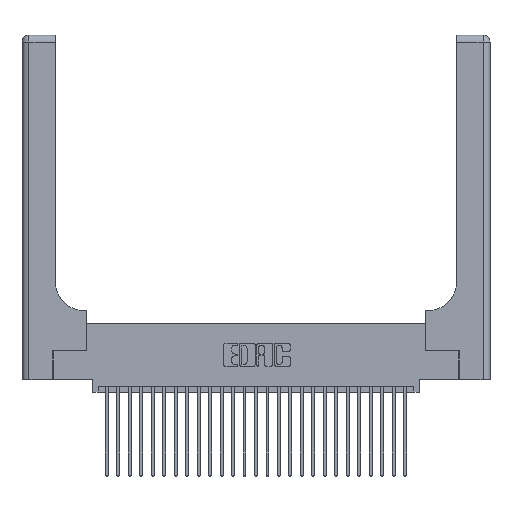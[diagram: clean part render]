
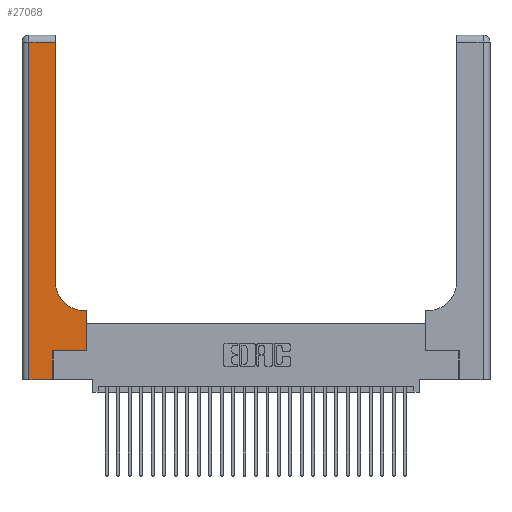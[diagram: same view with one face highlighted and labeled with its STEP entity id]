
A CAD part, top view. The second image highlights one B-rep face of the part: STEP entity #27068.
In plain terms, the highlighted planar face has unit normal (0, 0, 1).
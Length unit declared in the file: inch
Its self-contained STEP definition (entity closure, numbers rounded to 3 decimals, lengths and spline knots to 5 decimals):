
#70 = DIRECTION ( 'NONE',  ( 0., 1., 0. ) ) ;
#232 = DIRECTION ( 'NONE',  ( -1., 0., 0. ) ) ;
#331 = LINE ( 'NONE', #8050, #4463 ) ;
#711 = CARTESIAN_POINT ( 'NONE',  ( 0.2915, 3., 0.37 ) ) ;
#881 = ORIENTED_EDGE ( 'NONE', *, *, #12145, .T. ) ;
#1142 = VERTEX_POINT ( 'NONE', #8361 ) ;
#1199 = VERTEX_POINT ( 'NONE', #6777 ) ;
#1335 = ORIENTED_EDGE ( 'NONE', *, *, #14976, .T. ) ;
#1405 = VERTEX_POINT ( 'NONE', #6571 ) ;
#1464 = ORIENTED_EDGE ( 'NONE', *, *, #23641, .T. ) ;
#1806 = DIRECTION ( 'NONE',  ( 1., 0., 0. ) ) ;
#2013 = CARTESIAN_POINT ( 'NONE',  ( 0.5415, 0.85, 0.37 ) ) ;
#2093 = LINE ( 'NONE', #711, #17286 ) ;
#2987 = ORIENTED_EDGE ( 'NONE', *, *, #19149, .T. ) ;
#3297 = EDGE_CURVE ( 'NONE', #17739, #1199, #13120, .T. ) ;
#3792 = FACE_OUTER_BOUND ( 'NONE', #11331, .T. ) ;
#3968 = VECTOR ( 'NONE', #5839, 39.37008 ) ;
#4463 = VECTOR ( 'NONE', #28068, 39.37008 ) ;
#4515 = CARTESIAN_POINT ( 'NONE',  ( 0.269, 0., 0.37 ) ) ;
#4534 = EDGE_CURVE ( 'NONE', #8665, #1142, #23366, .T. ) ;
#4782 = PLANE ( 'NONE',  #22796 ) ;
#4822 = VECTOR ( 'NONE', #16466, 39.37008 ) ;
#5832 = CARTESIAN_POINT ( 'NONE',  ( 0.2915, 0.6, 0.37 ) ) ;
#5839 = DIRECTION ( 'NONE',  ( -1., 0., 0. ) ) ;
#5978 = VECTOR ( 'NONE', #22544, 39.37008 ) ;
#6223 = LINE ( 'NONE', #26571, #25215 ) ;
#6312 = LINE ( 'NONE', #5832, #12573 ) ;
#6571 = CARTESIAN_POINT ( 'NONE',  ( 0.2915, 2.94, 0.37 ) ) ;
#6777 = CARTESIAN_POINT ( 'NONE',  ( 0.5585, 0.25, 0.37 ) ) ;
#7262 = EDGE_CURVE ( 'NONE', #9841, #19209, #14631, .T. ) ;
#8050 = CARTESIAN_POINT ( 'NONE',  ( 0., 0., 0.37 ) ) ;
#8144 = LINE ( 'NONE', #19486, #3968 ) ;
#8361 = CARTESIAN_POINT ( 'NONE',  ( 0.2915, 0.85, 0.37 ) ) ;
#8665 = VERTEX_POINT ( 'NONE', #24727 ) ;
#8831 = DIRECTION ( 'NONE',  ( 0., 1., 0. ) ) ;
#9298 = AXIS2_PLACEMENT_3D ( 'NONE', #2013, #13096, #1806 ) ;
#9841 = VERTEX_POINT ( 'NONE', #17469 ) ;
#10858 = EDGE_CURVE ( 'NONE', #1405, #9841, #8144, .T. ) ;
#11331 = EDGE_LOOP ( 'NONE', ( #1335, #15556, #21869, #14901, #1464, #16745, #2987, #881, #26623 ) ) ;
#12145 = EDGE_CURVE ( 'NONE', #14466, #8665, #6312, .T. ) ;
#12573 = VECTOR ( 'NONE', #27729, 39.37008 ) ;
#13096 = DIRECTION ( 'NONE',  ( 0., 0., -1. ) ) ;
#13120 = LINE ( 'NONE', #16359, #4822 ) ;
#13189 = CARTESIAN_POINT ( 'NONE',  ( 0.06, 0., 0.37 ) ) ;
#13396 = CARTESIAN_POINT ( 'NONE',  ( 0., 3., 0.37 ) ) ;
#14466 = VERTEX_POINT ( 'NONE', #15961 ) ;
#14631 = LINE ( 'NONE', #18017, #5978 ) ;
#14901 = ORIENTED_EDGE ( 'NONE', *, *, #27447, .T. ) ;
#14976 = EDGE_CURVE ( 'NONE', #1142, #1405, #2093, .T. ) ;
#15240 = CARTESIAN_POINT ( 'NONE',  ( 0.269, 0., 0.37 ) ) ;
#15556 = ORIENTED_EDGE ( 'NONE', *, *, #10858, .T. ) ;
#15611 = DIRECTION ( 'NONE',  ( 0., 0., -1. ) ) ;
#15961 = CARTESIAN_POINT ( 'NONE',  ( 0.5585, 0.6, 0.37 ) ) ;
#16359 = CARTESIAN_POINT ( 'NONE',  ( 0.269, 0.25, 0.37 ) ) ;
#16466 = DIRECTION ( 'NONE',  ( 1., 0., 0. ) ) ;
#16745 = ORIENTED_EDGE ( 'NONE', *, *, #3297, .T. ) ;
#17286 = VECTOR ( 'NONE', #18497, 39.37008 ) ;
#17469 = CARTESIAN_POINT ( 'NONE',  ( 0.06, 2.94, 0.37 ) ) ;
#17739 = VERTEX_POINT ( 'NONE', #19750 ) ;
#18017 = CARTESIAN_POINT ( 'NONE',  ( 0.06, 3., 0.37 ) ) ;
#18497 = DIRECTION ( 'NONE',  ( 0., 1., 0. ) ) ;
#19149 = EDGE_CURVE ( 'NONE', #1199, #14466, #6223, .T. ) ;
#19181 = VECTOR ( 'NONE', #70, 39.37008 ) ;
#19209 = VERTEX_POINT ( 'NONE', #13189 ) ;
#19486 = CARTESIAN_POINT ( 'NONE',  ( 0., 2.94, 0.37 ) ) ;
#19750 = CARTESIAN_POINT ( 'NONE',  ( 0.269, 0.25, 0.37 ) ) ;
#21869 = ORIENTED_EDGE ( 'NONE', *, *, #7262, .T. ) ;
#22544 = DIRECTION ( 'NONE',  ( 0., -1., 0. ) ) ;
#22796 = AXIS2_PLACEMENT_3D ( 'NONE', #13396, #15611, #232 ) ;
#23366 = CIRCLE ( 'NONE', #9298, 0.25 ) ;
#23641 = EDGE_CURVE ( 'NONE', #28526, #17739, #26749, .T. ) ;
#24727 = CARTESIAN_POINT ( 'NONE',  ( 0.5415, 0.6, 0.37 ) ) ;
#25215 = VECTOR ( 'NONE', #8831, 39.37008 ) ;
#26571 = CARTESIAN_POINT ( 'NONE',  ( 0.5585, 0.25, 0.37 ) ) ;
#26623 = ORIENTED_EDGE ( 'NONE', *, *, #4534, .T. ) ;
#26749 = LINE ( 'NONE', #4515, #19181 ) ;
#27068 = ADVANCED_FACE ( 'NONE', ( #3792 ), #4782, .F. ) ;
#27447 = EDGE_CURVE ( 'NONE', #19209, #28526, #331, .T. ) ;
#27729 = DIRECTION ( 'NONE',  ( -1., 0., 0. ) ) ;
#28068 = DIRECTION ( 'NONE',  ( 1., 0., 0. ) ) ;
#28526 = VERTEX_POINT ( 'NONE', #15240 ) ;
